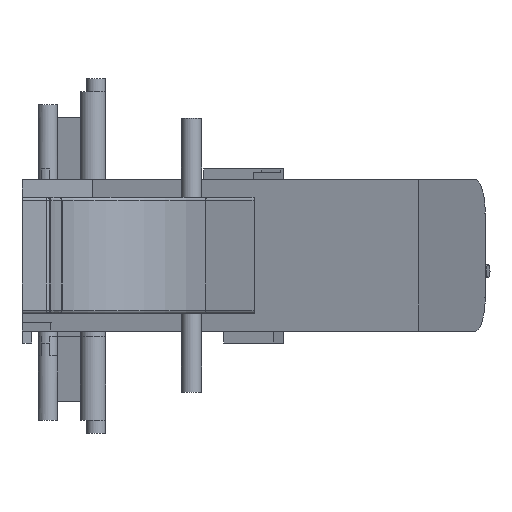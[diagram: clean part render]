
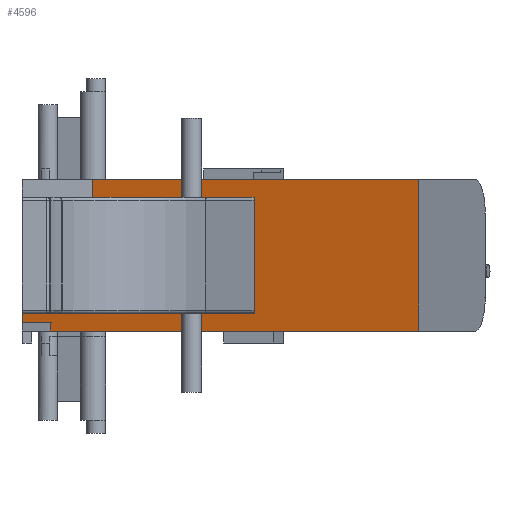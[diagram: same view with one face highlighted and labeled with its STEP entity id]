
A CAD part, left-side view. The second image highlights one B-rep face of the part: STEP entity #4596.
In plain terms, the highlighted planar face has unit normal (-0.951, 0.309, 0).
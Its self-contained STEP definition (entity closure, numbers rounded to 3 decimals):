
#615=FACE_OUTER_BOUND('',#880,.T.);
#880=EDGE_LOOP('',(#4194,#4195,#4196,#4197,#4198,#4199,#4200,#4201));
#919=LINE('',#6369,#1350);
#940=LINE('',#6429,#1371);
#1098=LINE('',#7707,#1529);
#1106=LINE('',#7722,#1537);
#1149=LINE('',#7827,#1580);
#1157=LINE('',#7842,#1588);
#1346=LINE('',#9021,#1777);
#1349=LINE('',#9030,#1780);
#1350=VECTOR('',#5056,10.);
#1371=VECTOR('',#5101,10.);
#1529=VECTOR('',#5603,10.);
#1537=VECTOR('',#5615,10.);
#1580=VECTOR('',#5712,10.);
#1588=VECTOR('',#5730,10.);
#1777=VECTOR('',#6349,10.);
#1780=VECTOR('',#6362,10.);
#1781=VERTEX_POINT('',#6367);
#1782=VERTEX_POINT('',#6368);
#1806=VERTEX_POINT('',#6427);
#1979=VERTEX_POINT('',#7705);
#1980=VERTEX_POINT('',#7706);
#1985=VERTEX_POINT('',#7720);
#2017=VERTEX_POINT('',#7825);
#2019=VERTEX_POINT('',#7840);
#2201=EDGE_CURVE('',#1781,#1782,#919,.T.);
#2230=EDGE_CURVE('',#1806,#1781,#940,.T.);
#2482=EDGE_CURVE('',#1979,#1980,#1098,.T.);
#2490=EDGE_CURVE('',#1980,#1985,#1106,.T.);
#2543=EDGE_CURVE('',#1806,#2017,#1149,.T.);
#2551=EDGE_CURVE('',#2017,#2019,#1157,.T.);
#2866=EDGE_CURVE('',#2019,#1979,#1346,.T.);
#2871=EDGE_CURVE('',#1782,#1985,#1349,.T.);
#4194=ORIENTED_EDGE('',*,*,#2230,.F.);
#4195=ORIENTED_EDGE('',*,*,#2543,.T.);
#4196=ORIENTED_EDGE('',*,*,#2551,.T.);
#4197=ORIENTED_EDGE('',*,*,#2866,.T.);
#4198=ORIENTED_EDGE('',*,*,#2482,.T.);
#4199=ORIENTED_EDGE('',*,*,#2490,.T.);
#4200=ORIENTED_EDGE('',*,*,#2871,.F.);
#4201=ORIENTED_EDGE('',*,*,#2201,.F.);
#4337=PLANE('',#5050);
#4596=ADVANCED_FACE('',(#615),#4337,.T.);
#5050=AXIS2_PLACEMENT_3D('',#9029,#6360,#6361);
#5056=DIRECTION('',(0.,0.,-1.));
#5101=DIRECTION('',(-0.309,-0.951,0.));
#5603=DIRECTION('',(-0.309,-0.951,0.));
#5615=DIRECTION('',(0.,0.,-1.));
#5712=DIRECTION('',(0.,0.,-1.));
#5730=DIRECTION('',(0.309,0.951,0.));
#6349=DIRECTION('',(0.,0.,-1.));
#6360=DIRECTION('center_axis',(-0.951,0.309,0.));
#6361=DIRECTION('ref_axis',(0.,0.,
1.));
#6362=DIRECTION('',(0.309,0.951,0.));
#6367=CARTESIAN_POINT('',(13.591,-63.052,11.75));
#6368=CARTESIAN_POINT('',(13.591,-63.052,-11.75));
#6369=CARTESIAN_POINT('',(13.591,-63.052,-5.875));
#6427=CARTESIAN_POINT('',(30.049,-12.4,11.75));
#6429=CARTESIAN_POINT('',(2.312,-97.765,11.75));
#7705=CARTESIAN_POINT('',(33.591,-1.5,-10.375));
#7706=CARTESIAN_POINT('',(32.169,-5.875,-10.375));
#7707=CARTESIAN_POINT('',(17.241,-51.82,-10.375));
#7720=CARTESIAN_POINT('',(32.169,-5.875,-11.75));
#7722=CARTESIAN_POINT('',(32.169,-5.875,-5.875));
#7825=CARTESIAN_POINT('',(30.049,-12.4,4.75));
#7827=CARTESIAN_POINT('',(30.049,-12.4,2.982));
#7840=CARTESIAN_POINT('',(33.591,-1.5,4.75));
#7842=CARTESIAN_POINT('',(18.86,-46.836,4.75));
#9021=CARTESIAN_POINT('',(33.591,-1.5,-5.875));
#9029=CARTESIAN_POINT('Origin',(2.312,-97.765,-11.75));
#9030=CARTESIAN_POINT('',(2.312,-97.765,-11.75));
